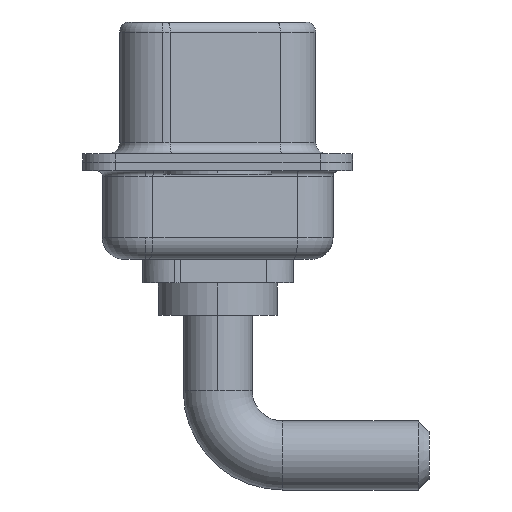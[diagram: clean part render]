
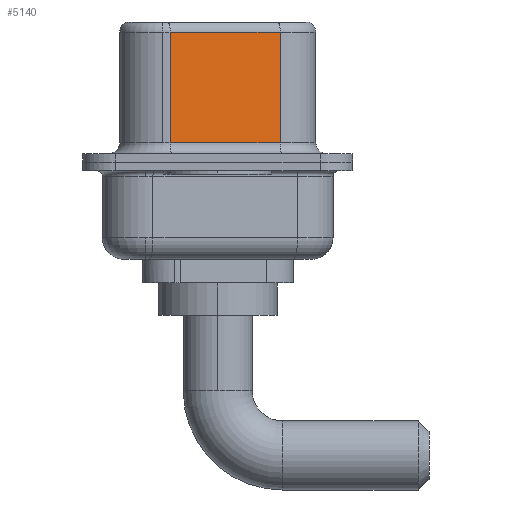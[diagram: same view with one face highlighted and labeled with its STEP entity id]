
A CAD part, left-side view. The second image highlights one B-rep face of the part: STEP entity #5140.
In plain terms, the highlighted planar face has unit normal (-0.985, -0.174, 0).
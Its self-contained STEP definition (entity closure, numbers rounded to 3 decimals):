
#82 = CARTESIAN_POINT ( 'NONE',  ( 4.58, -2.897, 6.52 ) ) ;
#284 = ORIENTED_EDGE ( 'NONE', *, *, #2141, .T. ) ;
#335 = AXIS2_PLACEMENT_3D ( 'NONE', #82, #3933, #6912 ) ;
#673 = CARTESIAN_POINT ( 'NONE',  ( 4.58, -2.897, 6.52 ) ) ;
#788 = ORIENTED_EDGE ( 'NONE', *, *, #6591, .T. ) ;
#1359 = CARTESIAN_POINT ( 'NONE',  ( 4.58, -2.897, 6.02 ) ) ;
#1364 = VECTOR ( 'NONE', #11095, 1000. ) ;
#1831 = LINE ( 'NONE', #6724, #9725 ) ;
#2141 = EDGE_CURVE ( 'NONE', #6054, #3684, #3486, .T. ) ;
#2168 = EDGE_CURVE ( 'NONE', #3363, #5488, #3547, .T. ) ;
#2272 = VECTOR ( 'NONE', #2665, 1000. ) ;
#2641 = CARTESIAN_POINT ( 'NONE',  ( 4.58, -2.897, 0.9 ) ) ;
#2665 = DIRECTION ( 'NONE',  ( 0., 0., -1. ) ) ;
#2893 = VECTOR ( 'NONE', #12317, 1000. ) ;
#3363 = VERTEX_POINT ( 'NONE', #11362 ) ;
#3486 = LINE ( 'NONE', #4445, #2893 ) ;
#3547 = LINE ( 'NONE', #673, #2272 ) ;
#3684 = VERTEX_POINT ( 'NONE', #9273 ) ;
#3933 = DIRECTION ( 'NONE',  ( 0.985, 0.174, 0. ) ) ;
#4361 = LINE ( 'NONE', #1359, #1364 ) ;
#4365 = EDGE_LOOP ( 'NONE', ( #9023, #788, #284, #7399 ) ) ;
#4445 = CARTESIAN_POINT ( 'NONE',  ( 3.68, 2.203, 6.52 ) ) ;
#4848 = CARTESIAN_POINT ( 'NONE',  ( 3.68, 2.203, 6.02 ) ) ;
#5087 = EDGE_CURVE ( 'NONE', #3684, #5488, #1831, .T. ) ;
#5140 = ADVANCED_FACE ( 'NONE', ( #10732 ), #11684, .F. ) ;
#5488 = VERTEX_POINT ( 'NONE', #2641 ) ;
#5640 = DIRECTION ( 'NONE',  ( 0.174, -0.985, 0. ) ) ;
#6054 = VERTEX_POINT ( 'NONE', #4848 ) ;
#6591 = EDGE_CURVE ( 'NONE', #3363, #6054, #4361, .T. ) ;
#6724 = CARTESIAN_POINT ( 'NONE',  ( 4.58, -2.897, 0.9 ) ) ;
#6912 = DIRECTION ( 'NONE',  ( -0.174, 0.985, 0. ) ) ;
#7399 = ORIENTED_EDGE ( 'NONE', *, *, #5087, .T. ) ;
#9023 = ORIENTED_EDGE ( 'NONE', *, *, #2168, .F. ) ;
#9273 = CARTESIAN_POINT ( 'NONE',  ( 3.68, 2.203, 0.9 ) ) ;
#9725 = VECTOR ( 'NONE', #5640, 1000. ) ;
#10732 = FACE_OUTER_BOUND ( 'NONE', #4365, .T. ) ;
#11095 = DIRECTION ( 'NONE',  ( -0.174, 0.985, 0. ) ) ;
#11362 = CARTESIAN_POINT ( 'NONE',  ( 4.58, -2.897, 6.02 ) ) ;
#11684 = PLANE ( 'NONE',  #335 ) ;
#12317 = DIRECTION ( 'NONE',  ( 0., 0., -1. ) ) ;
